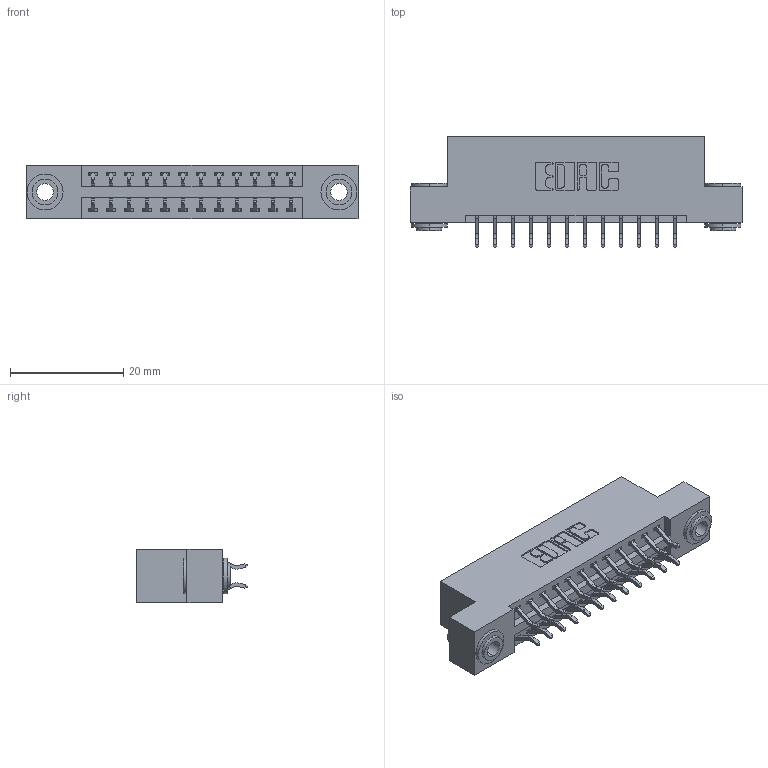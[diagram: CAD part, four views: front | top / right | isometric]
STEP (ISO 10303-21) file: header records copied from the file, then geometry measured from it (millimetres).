
FILE_DESCRIPTION (( 'STEP AP203' ), '1' );
FILE_NAME ('396-024-556-203.STEP', '2019-10-30T04:25:13', ( '' ), ( '' ), 'SwSTEP 2.0', 'SolidWorks 2016', '' );
FILE_SCHEMA (( 'CONFIG_CONTROL_DESIGN' ));
Length unit declared in the file: inch
Products named in the file (4): 346 Part_Flush Mounting Lugs - 0.156 Dia-TH; 396-024-556-203; 345-250-002_345-250-002-102; 345-292-001_556 Tail
Assembly tree (27 placements, depth 2):
  396-024-556-203
    346 Part_Flush Mounting Lugs - 0.156 Dia-TH
    345-292-001_556 Tail  x24
    345-250-002_345-250-002-102  x2
Bounding box: 58.67 x 19.57 x 9.4 mm (x, y, z)
Volume: 5506.9 mm3; surface area: 7289.9 mm2
Topology: 27 solids, 27 shells, 1552 faces, 4557 edges, 3002 vertices
Faces by surface type: plane 1022, cylinder 522, cone 8
Entity records: 12740 total; most frequent: CARTESIAN_POINT 2131, ORIENTED_EDGE 2046, DIRECTION 1949, EDGE_CURVE 1023, LINE 811, VECTOR 811, VERTEX_POINT 678, AXIS2_PLACEMENT_3D 569
